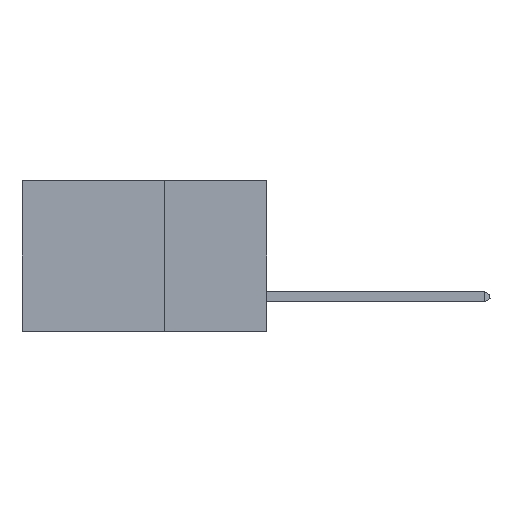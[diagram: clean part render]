
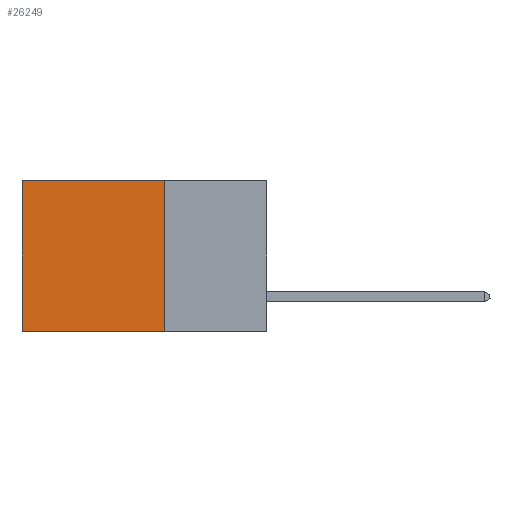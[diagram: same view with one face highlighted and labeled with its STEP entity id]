
A CAD part, left-side view. The second image highlights one B-rep face of the part: STEP entity #26249.
In plain terms, the highlighted planar face has unit normal (-1, 0, 0).
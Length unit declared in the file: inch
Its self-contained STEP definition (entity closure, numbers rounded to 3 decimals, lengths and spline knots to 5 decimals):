
#471 = EDGE_CURVE ( 'NONE', #18186, #20664, #9020, .T. ) ;
#843 = VECTOR ( 'NONE', #16255, 39.37008 ) ;
#2487 = EDGE_CURVE ( 'NONE', #22728, #20664, #4249, .T. ) ;
#2624 = DIRECTION ( 'NONE',  ( 0., 0., -1. ) ) ;
#4249 = LINE ( 'NONE', #15232, #11833 ) ;
#5135 = CARTESIAN_POINT ( 'NONE',  ( 0.2875, 0.6, 0. ) ) ;
#5668 = DIRECTION ( 'NONE',  ( 0., 0., -1. ) ) ;
#5762 = CARTESIAN_POINT ( 'NONE',  ( 0.2875, 0.25, 0. ) ) ;
#6061 = LINE ( 'NONE', #22988, #26454 ) ;
#6656 = CARTESIAN_POINT ( 'NONE',  ( 0.2875, 0.6, 0. ) ) ;
#9020 = LINE ( 'NONE', #6656, #12655 ) ;
#9721 = EDGE_CURVE ( 'NONE', #22579, #18186, #13724, .T. ) ;
#10033 = DIRECTION ( 'NONE',  ( 0., 0., -1. ) ) ;
#10406 = ORIENTED_EDGE ( 'NONE', *, *, #9721, .T. ) ;
#11833 = VECTOR ( 'NONE', #19741, 39.37008 ) ;
#11963 = ORIENTED_EDGE ( 'NONE', *, *, #471, .T. ) ;
#12038 = DIRECTION ( 'NONE',  ( 1., 0., 0. ) ) ;
#12186 = ORIENTED_EDGE ( 'NONE', *, *, #2487, .F. ) ;
#12655 = VECTOR ( 'NONE', #2624, 39.37008 ) ;
#13724 = LINE ( 'NONE', #26720, #843 ) ;
#15232 = CARTESIAN_POINT ( 'NONE',  ( 0.2875, 0.25, -0.37 ) ) ;
#16255 = DIRECTION ( 'NONE',  ( 0., 1., 0. ) ) ;
#17382 = CARTESIAN_POINT ( 'NONE',  ( 0.2875, 0.6, -0.37 ) ) ;
#17833 = EDGE_CURVE ( 'NONE', #22579, #22728, #6061, .T. ) ;
#18186 = VERTEX_POINT ( 'NONE', #5135 ) ;
#18377 = PLANE ( 'NONE',  #21739 ) ;
#19741 = DIRECTION ( 'NONE',  ( 0., 1., 0. ) ) ;
#20613 = FACE_OUTER_BOUND ( 'NONE', #21411, .T. ) ;
#20664 = VERTEX_POINT ( 'NONE', #17382 ) ;
#20989 = CARTESIAN_POINT ( 'NONE',  ( 0.2875, 0.25, -0.37 ) ) ;
#21411 = EDGE_LOOP ( 'NONE', ( #11963, #12186, #24675, #10406 ) ) ;
#21739 = AXIS2_PLACEMENT_3D ( 'NONE', #5762, #12038, #5668 ) ;
#22235 = CARTESIAN_POINT ( 'NONE',  ( 0.2875, 0.25, 0. ) ) ;
#22579 = VERTEX_POINT ( 'NONE', #22235 ) ;
#22728 = VERTEX_POINT ( 'NONE', #20989 ) ;
#22988 = CARTESIAN_POINT ( 'NONE',  ( 0.2875, 0.25, 0. ) ) ;
#24675 = ORIENTED_EDGE ( 'NONE', *, *, #17833, .F. ) ;
#26249 = ADVANCED_FACE ( 'NONE', ( #20613 ), #18377, .F. ) ;
#26454 = VECTOR ( 'NONE', #10033, 39.37008 ) ;
#26720 = CARTESIAN_POINT ( 'NONE',  ( 0.2875, 0.25, 0. ) ) ;
